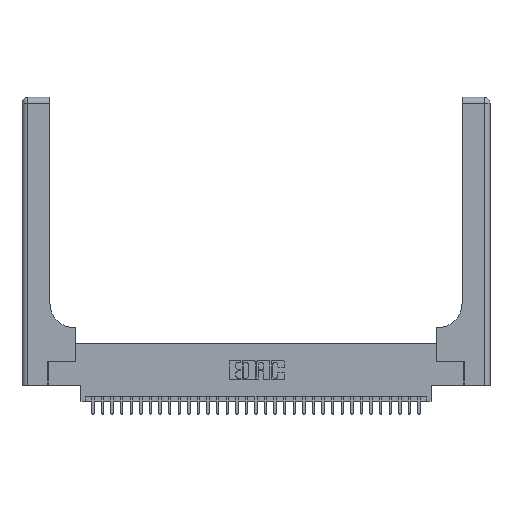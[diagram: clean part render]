
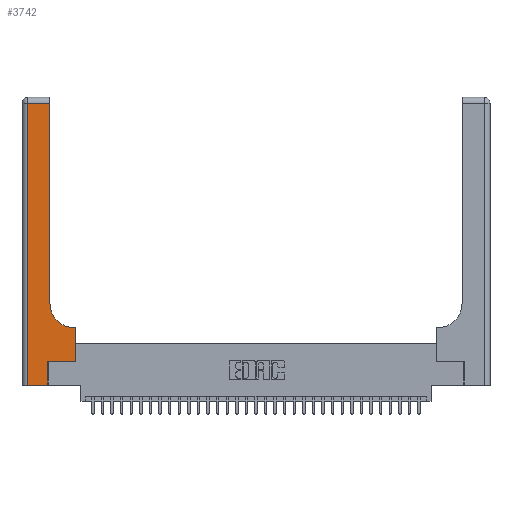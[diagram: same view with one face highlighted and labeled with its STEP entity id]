
A CAD part, top view. The second image highlights one B-rep face of the part: STEP entity #3742.
In plain terms, the highlighted planar face has unit normal (0, 0, 1).
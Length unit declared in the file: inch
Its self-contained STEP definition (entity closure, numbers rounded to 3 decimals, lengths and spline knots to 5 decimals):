
#154 = CIRCLE ( 'NONE', #940, 0.25 ) ;
#216 = CARTESIAN_POINT ( 'NONE',  ( 0.06, 0., 0.37 ) ) ;
#574 = CARTESIAN_POINT ( 'NONE',  ( 0.269, 0.25, 0.37 ) ) ;
#630 = CARTESIAN_POINT ( 'NONE',  ( 0.5415, 0.85, 0.37 ) ) ;
#666 = VERTEX_POINT ( 'NONE', #29484 ) ;
#940 = AXIS2_PLACEMENT_3D ( 'NONE', #630, #28904, #11045 ) ;
#1276 = CARTESIAN_POINT ( 'NONE',  ( 0., 3., 0.37 ) ) ;
#1636 = DIRECTION ( 'NONE',  ( -1., 0., 0. ) ) ;
#2218 = VERTEX_POINT ( 'NONE', #21402 ) ;
#2477 = VERTEX_POINT ( 'NONE', #11969 ) ;
#3004 = ORIENTED_EDGE ( 'NONE', *, *, #9461, .T. ) ;
#3742 = ADVANCED_FACE ( 'NONE', ( #23852 ), #11672, .F. ) ;
#3931 = CARTESIAN_POINT ( 'NONE',  ( 0.269, 0.25, 0.37 ) ) ;
#4129 = VECTOR ( 'NONE', #15295, 39.37008 ) ;
#4221 = ORIENTED_EDGE ( 'NONE', *, *, #32010, .T. ) ;
#4415 = VERTEX_POINT ( 'NONE', #574 ) ;
#4675 = VECTOR ( 'NONE', #22168, 39.37008 ) ;
#5672 = EDGE_CURVE ( 'NONE', #4415, #2218, #6297, .T. ) ;
#6297 = LINE ( 'NONE', #3931, #4675 ) ;
#7037 = VECTOR ( 'NONE', #20326, 39.37008 ) ;
#7206 = CARTESIAN_POINT ( 'NONE',  ( 0., 2.94, 0.37 ) ) ;
#7668 = VECTOR ( 'NONE', #1636, 39.37008 ) ;
#8939 = LINE ( 'NONE', #9516, #21186 ) ;
#9292 = DIRECTION ( 'NONE',  ( 1., 0., 0. ) ) ;
#9461 = EDGE_CURVE ( 'NONE', #666, #14092, #27361, .T. ) ;
#9516 = CARTESIAN_POINT ( 'NONE',  ( 0., 0., 0.37 ) ) ;
#10497 = VECTOR ( 'NONE', #16162, 39.37008 ) ;
#10685 = DIRECTION ( 'NONE',  ( -1., 0., 0. ) ) ;
#11045 = DIRECTION ( 'NONE',  ( 1., 0., 0. ) ) ;
#11672 = PLANE ( 'NONE',  #26687 ) ;
#11969 = CARTESIAN_POINT ( 'NONE',  ( 0.269, 0., 0.37 ) ) ;
#12179 = VERTEX_POINT ( 'NONE', #18561 ) ;
#12616 = DIRECTION ( 'NONE',  ( 0., 1., 0. ) ) ;
#12643 = CARTESIAN_POINT ( 'NONE',  ( 0.5585, 0.25, 0.37 ) ) ;
#14005 = ORIENTED_EDGE ( 'NONE', *, *, #27340, .T. ) ;
#14092 = VERTEX_POINT ( 'NONE', #22701 ) ;
#15049 = CARTESIAN_POINT ( 'NONE',  ( 0.2915, 3., 0.37 ) ) ;
#15295 = DIRECTION ( 'NONE',  ( 0., 1., 0. ) ) ;
#15724 = CARTESIAN_POINT ( 'NONE',  ( 0.2915, 0.6, 0.37 ) ) ;
#15856 = VERTEX_POINT ( 'NONE', #216 ) ;
#15894 = VERTEX_POINT ( 'NONE', #33600 ) ;
#15916 = ORIENTED_EDGE ( 'NONE', *, *, #19146, .T. ) ;
#16162 = DIRECTION ( 'NONE',  ( 0., -1., 0. ) ) ;
#16609 = DIRECTION ( 'NONE',  ( -1., 0., 0. ) ) ;
#17958 = EDGE_CURVE ( 'NONE', #12179, #15856, #28404, .T. ) ;
#18561 = CARTESIAN_POINT ( 'NONE',  ( 0.06, 2.94, 0.37 ) ) ;
#19010 = ORIENTED_EDGE ( 'NONE', *, *, #26696, .T. ) ;
#19146 = EDGE_CURVE ( 'NONE', #21202, #666, #154, .T. ) ;
#19550 = DIRECTION ( 'NONE',  ( 0., 0., -1. ) ) ;
#20082 = VECTOR ( 'NONE', #12616, 39.37008 ) ;
#20326 = DIRECTION ( 'NONE',  ( 0., 1., 0. ) ) ;
#20506 = EDGE_CURVE ( 'NONE', #2477, #4415, #31461, .T. ) ;
#20568 = EDGE_LOOP ( 'NONE', ( #3004, #14005, #30595, #19010, #32748, #27319, #4221, #31581, #15916 ) ) ;
#21186 = VECTOR ( 'NONE', #9292, 39.37008 ) ;
#21202 = VERTEX_POINT ( 'NONE', #25822 ) ;
#21402 = CARTESIAN_POINT ( 'NONE',  ( 0.5585, 0.25, 0.37 ) ) ;
#21562 = LINE ( 'NONE', #15724, #29667 ) ;
#21674 = LINE ( 'NONE', #12643, #4129 ) ;
#22168 = DIRECTION ( 'NONE',  ( 1., 0., 0. ) ) ;
#22701 = CARTESIAN_POINT ( 'NONE',  ( 0.2915, 2.94, 0.37 ) ) ;
#23068 = EDGE_CURVE ( 'NONE', #15894, #21202, #21562, .T. ) ;
#23852 = FACE_OUTER_BOUND ( 'NONE', #20568, .T. ) ;
#25306 = CARTESIAN_POINT ( 'NONE',  ( 0.269, 0., 0.37 ) ) ;
#25822 = CARTESIAN_POINT ( 'NONE',  ( 0.5415, 0.6, 0.37 ) ) ;
#26687 = AXIS2_PLACEMENT_3D ( 'NONE', #1276, #19550, #16609 ) ;
#26696 = EDGE_CURVE ( 'NONE', #15856, #2477, #8939, .T. ) ;
#27319 = ORIENTED_EDGE ( 'NONE', *, *, #5672, .T. ) ;
#27340 = EDGE_CURVE ( 'NONE', #14092, #12179, #30471, .T. ) ;
#27361 = LINE ( 'NONE', #15049, #20082 ) ;
#28404 = LINE ( 'NONE', #31598, #10497 ) ;
#28904 = DIRECTION ( 'NONE',  ( 0., 0., -1. ) ) ;
#29484 = CARTESIAN_POINT ( 'NONE',  ( 0.2915, 0.85, 0.37 ) ) ;
#29667 = VECTOR ( 'NONE', #10685, 39.37008 ) ;
#30471 = LINE ( 'NONE', #7206, #7668 ) ;
#30595 = ORIENTED_EDGE ( 'NONE', *, *, #17958, .T. ) ;
#31461 = LINE ( 'NONE', #25306, #7037 ) ;
#31581 = ORIENTED_EDGE ( 'NONE', *, *, #23068, .T. ) ;
#31598 = CARTESIAN_POINT ( 'NONE',  ( 0.06, 3., 0.37 ) ) ;
#32010 = EDGE_CURVE ( 'NONE', #2218, #15894, #21674, .T. ) ;
#32748 = ORIENTED_EDGE ( 'NONE', *, *, #20506, .T. ) ;
#33600 = CARTESIAN_POINT ( 'NONE',  ( 0.5585, 0.6, 0.37 ) ) ;
